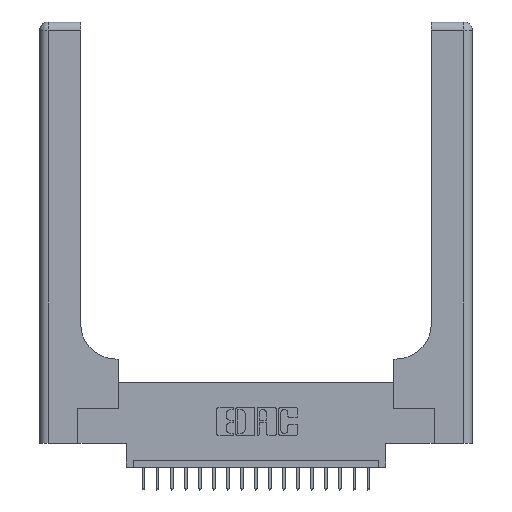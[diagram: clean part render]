
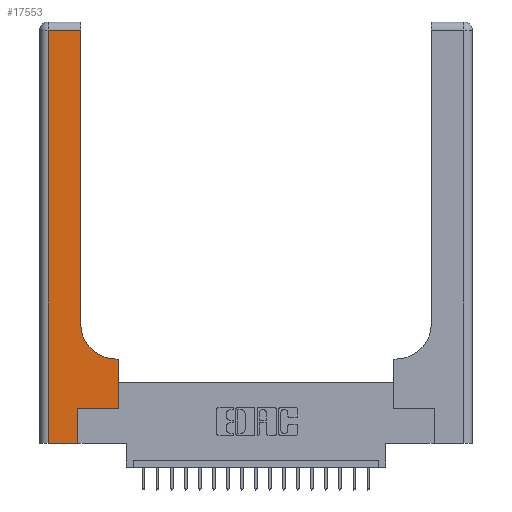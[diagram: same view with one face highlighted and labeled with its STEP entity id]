
A CAD part, top view. The second image highlights one B-rep face of the part: STEP entity #17553.
In plain terms, the highlighted planar face has unit normal (0, 0, 1).
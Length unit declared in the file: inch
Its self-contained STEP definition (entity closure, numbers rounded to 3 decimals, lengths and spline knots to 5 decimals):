
#475 = VERTEX_POINT ( 'NONE', #17163 ) ;
#579 = CARTESIAN_POINT ( 'NONE',  ( 0., 3., 0.37 ) ) ;
#912 = CARTESIAN_POINT ( 'NONE',  ( 0.5415, 0.85, 0.37 ) ) ;
#1042 = EDGE_CURVE ( 'NONE', #8612, #1074, #18863, .T. ) ;
#1074 = VERTEX_POINT ( 'NONE', #11353 ) ;
#1337 = CARTESIAN_POINT ( 'NONE',  ( 0.269, 0., 0.37 ) ) ;
#1457 = VECTOR ( 'NONE', #16211, 39.37008 ) ;
#2206 = VECTOR ( 'NONE', #4647, 39.37008 ) ;
#2515 = AXIS2_PLACEMENT_3D ( 'NONE', #912, #7556, #9222 ) ;
#3143 = ORIENTED_EDGE ( 'NONE', *, *, #1042, .T. ) ;
#3463 = CARTESIAN_POINT ( 'NONE',  ( 0.2915, 0.85, 0.37 ) ) ;
#3567 = ORIENTED_EDGE ( 'NONE', *, *, #14940, .T. ) ;
#3682 = DIRECTION ( 'NONE',  ( 0., -1., 0. ) ) ;
#4486 = EDGE_CURVE ( 'NONE', #475, #10720, #16332, .T. ) ;
#4519 = EDGE_CURVE ( 'NONE', #15792, #13728, #13189, .T. ) ;
#4576 = VECTOR ( 'NONE', #16628, 39.37008 ) ;
#4647 = DIRECTION ( 'NONE',  ( 0., 1., 0. ) ) ;
#5611 = LINE ( 'NONE', #21449, #4576 ) ;
#5676 = DIRECTION ( 'NONE',  ( -1., 0., 0. ) ) ;
#5851 = VECTOR ( 'NONE', #14113, 39.37008 ) ;
#6559 = EDGE_CURVE ( 'NONE', #1074, #9096, #10785, .T. ) ;
#6648 = LINE ( 'NONE', #12937, #2206 ) ;
#6692 = ORIENTED_EDGE ( 'NONE', *, *, #19889, .T. ) ;
#7015 = CARTESIAN_POINT ( 'NONE',  ( 0.06, 0., 0.37 ) ) ;
#7556 = DIRECTION ( 'NONE',  ( 0., 0., -1. ) ) ;
#8271 = EDGE_LOOP ( 'NONE', ( #3567, #16727, #12915, #6692, #3143, #13319, #14704, #19514, #20978 ) ) ;
#8612 = VERTEX_POINT ( 'NONE', #20150 ) ;
#8865 = CARTESIAN_POINT ( 'NONE',  ( 0.2915, 0.6, 0.37 ) ) ;
#9096 = VERTEX_POINT ( 'NONE', #9920 ) ;
#9222 = DIRECTION ( 'NONE',  ( 1., 0., 0. ) ) ;
#9920 = CARTESIAN_POINT ( 'NONE',  ( 0.5585, 0.25, 0.37 ) ) ;
#10535 = CARTESIAN_POINT ( 'NONE',  ( 0.06, 3., 0.37 ) ) ;
#10720 = VERTEX_POINT ( 'NONE', #3463 ) ;
#10785 = LINE ( 'NONE', #21018, #5851 ) ;
#10926 = CARTESIAN_POINT ( 'NONE',  ( 0., 2.94, 0.37 ) ) ;
#11353 = CARTESIAN_POINT ( 'NONE',  ( 0.269, 0.25, 0.37 ) ) ;
#11368 = VECTOR ( 'NONE', #3682, 39.37008 ) ;
#12280 = PLANE ( 'NONE',  #15631 ) ;
#12292 = VECTOR ( 'NONE', #14270, 39.37008 ) ;
#12915 = ORIENTED_EDGE ( 'NONE', *, *, #4519, .T. ) ;
#12937 = CARTESIAN_POINT ( 'NONE',  ( 0.2915, 3., 0.37 ) ) ;
#13094 = EDGE_CURVE ( 'NONE', #16986, #475, #16589, .T. ) ;
#13189 = LINE ( 'NONE', #10535, #11368 ) ;
#13319 = ORIENTED_EDGE ( 'NONE', *, *, #6559, .T. ) ;
#13344 = VERTEX_POINT ( 'NONE', #21212 ) ;
#13485 = FACE_OUTER_BOUND ( 'NONE', #8271, .T. ) ;
#13525 = EDGE_CURVE ( 'NONE', #9096, #16986, #20229, .T. ) ;
#13625 = CARTESIAN_POINT ( 'NONE',  ( 0.5585, 0.25, 0.37 ) ) ;
#13728 = VERTEX_POINT ( 'NONE', #7015 ) ;
#14113 = DIRECTION ( 'NONE',  ( 1., 0., 0. ) ) ;
#14270 = DIRECTION ( 'NONE',  ( -1., 0., 0. ) ) ;
#14704 = ORIENTED_EDGE ( 'NONE', *, *, #13525, .T. ) ;
#14940 = EDGE_CURVE ( 'NONE', #10720, #13344, #6648, .T. ) ;
#15628 = EDGE_CURVE ( 'NONE', #13344, #15792, #16944, .T. ) ;
#15631 = AXIS2_PLACEMENT_3D ( 'NONE', #579, #17211, #5676 ) ;
#15792 = VERTEX_POINT ( 'NONE', #17960 ) ;
#15802 = VECTOR ( 'NONE', #16963, 39.37008 ) ;
#16211 = DIRECTION ( 'NONE',  ( 0., 1., 0. ) ) ;
#16332 = CIRCLE ( 'NONE', #2515, 0.25 ) ;
#16589 = LINE ( 'NONE', #8865, #17635 ) ;
#16628 = DIRECTION ( 'NONE',  ( 1., 0., 0. ) ) ;
#16727 = ORIENTED_EDGE ( 'NONE', *, *, #15628, .T. ) ;
#16944 = LINE ( 'NONE', #10926, #12292 ) ;
#16963 = DIRECTION ( 'NONE',  ( 0., 1., 0. ) ) ;
#16986 = VERTEX_POINT ( 'NONE', #21200 ) ;
#16993 = DIRECTION ( 'NONE',  ( -1., 0., 0. ) ) ;
#17163 = CARTESIAN_POINT ( 'NONE',  ( 0.5415, 0.6, 0.37 ) ) ;
#17211 = DIRECTION ( 'NONE',  ( 0., 0., -1. ) ) ;
#17553 = ADVANCED_FACE ( 'NONE', ( #13485 ), #12280, .F. ) ;
#17635 = VECTOR ( 'NONE', #16993, 39.37008 ) ;
#17960 = CARTESIAN_POINT ( 'NONE',  ( 0.06, 2.94, 0.37 ) ) ;
#18863 = LINE ( 'NONE', #1337, #1457 ) ;
#19514 = ORIENTED_EDGE ( 'NONE', *, *, #13094, .T. ) ;
#19889 = EDGE_CURVE ( 'NONE', #13728, #8612, #5611, .T. ) ;
#20150 = CARTESIAN_POINT ( 'NONE',  ( 0.269, 0., 0.37 ) ) ;
#20229 = LINE ( 'NONE', #13625, #15802 ) ;
#20978 = ORIENTED_EDGE ( 'NONE', *, *, #4486, .T. ) ;
#21018 = CARTESIAN_POINT ( 'NONE',  ( 0.269, 0.25, 0.37 ) ) ;
#21200 = CARTESIAN_POINT ( 'NONE',  ( 0.5585, 0.6, 0.37 ) ) ;
#21212 = CARTESIAN_POINT ( 'NONE',  ( 0.2915, 2.94, 0.37 ) ) ;
#21449 = CARTESIAN_POINT ( 'NONE',  ( 0., 0., 0.37 ) ) ;
